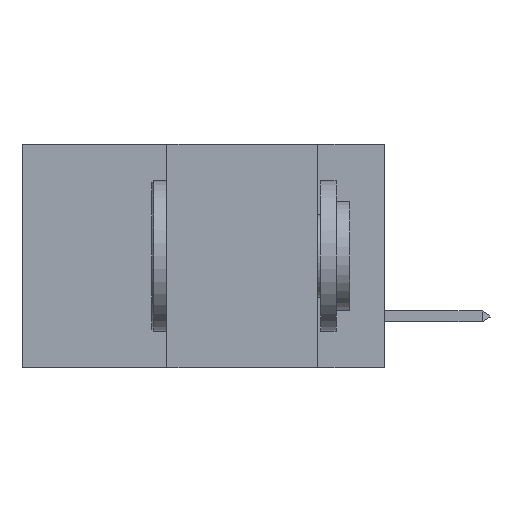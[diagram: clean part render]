
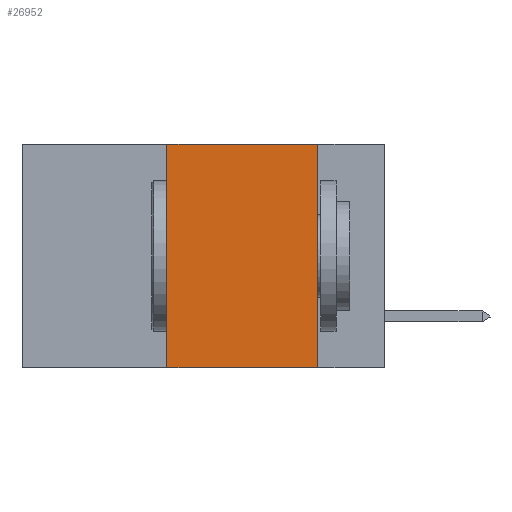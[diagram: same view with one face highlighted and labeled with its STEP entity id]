
A CAD part, left-side view. The second image highlights one B-rep face of the part: STEP entity #26952.
In plain terms, the highlighted planar face has unit normal (-1, 0, 0).
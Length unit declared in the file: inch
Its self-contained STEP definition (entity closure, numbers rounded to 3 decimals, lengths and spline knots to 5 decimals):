
#34 = EDGE_CURVE ( 'NONE', #44070, #2648, #2830, .T. ) ;
#351 = LINE ( 'NONE', #17322, #23861 ) ;
#598 = ORIENTED_EDGE ( 'NONE', *, *, #30831, .F. ) ;
#2648 = VERTEX_POINT ( 'NONE', #30350 ) ;
#2830 = LINE ( 'NONE', #42293, #42597 ) ;
#2924 = DIRECTION ( 'NONE',  ( 1., 0., 0. ) ) ;
#6303 = EDGE_CURVE ( 'NONE', #29232, #2648, #351, .T. ) ;
#7140 = DIRECTION ( 'NONE',  ( 0., 0., -1. ) ) ;
#9015 = ORIENTED_EDGE ( 'NONE', *, *, #34, .F. ) ;
#9149 = CARTESIAN_POINT ( 'NONE',  ( 0., 0.36, 0. ) ) ;
#11955 = FACE_OUTER_BOUND ( 'NONE', #38855, .T. ) ;
#13648 = CARTESIAN_POINT ( 'NONE',  ( 0., 0.36, 0. ) ) ;
#14920 = CARTESIAN_POINT ( 'NONE',  ( 0., 0.36, -0.37 ) ) ;
#17322 = CARTESIAN_POINT ( 'NONE',  ( 0., 0.6, -0.37 ) ) ;
#21343 = DIRECTION ( 'NONE',  ( 0., -1., 0. ) ) ;
#21453 = CARTESIAN_POINT ( 'NONE',  ( 0., 0.6, 0. ) ) ;
#22094 = PLANE ( 'NONE',  #35613 ) ;
#22651 = CARTESIAN_POINT ( 'NONE',  ( 0., 0.11, 0. ) ) ;
#23861 = VECTOR ( 'NONE', #21343, 39.37008 ) ;
#24878 = VECTOR ( 'NONE', #33259, 39.37008 ) ;
#25992 = CARTESIAN_POINT ( 'NONE',  ( 0., 0.6, 0. ) ) ;
#26289 = DIRECTION ( 'NONE',  ( 0., 0., -1. ) ) ;
#26952 = ADVANCED_FACE ( 'NONE', ( #11955 ), #22094, .F. ) ;
#29232 = VERTEX_POINT ( 'NONE', #14920 ) ;
#30350 = CARTESIAN_POINT ( 'NONE',  ( 0., 0.11, -0.37 ) ) ;
#30831 = EDGE_CURVE ( 'NONE', #39962, #44070, #35675, .T. ) ;
#31560 = ORIENTED_EDGE ( 'NONE', *, *, #6303, .T. ) ;
#31675 = VECTOR ( 'NONE', #33351, 39.37008 ) ;
#33259 = DIRECTION ( 'NONE',  ( 0., -1., 0. ) ) ;
#33351 = DIRECTION ( 'NONE',  ( 0., 0., 1. ) ) ;
#35613 = AXIS2_PLACEMENT_3D ( 'NONE', #25992, #2924, #7140 ) ;
#35675 = LINE ( 'NONE', #21453, #24878 ) ;
#36117 = ORIENTED_EDGE ( 'NONE', *, *, #40064, .F. ) ;
#38855 = EDGE_LOOP ( 'NONE', ( #9015, #598, #36117, #31560 ) ) ;
#39478 = LINE ( 'NONE', #13648, #31675 ) ;
#39962 = VERTEX_POINT ( 'NONE', #9149 ) ;
#40064 = EDGE_CURVE ( 'NONE', #29232, #39962, #39478, .T. ) ;
#42293 = CARTESIAN_POINT ( 'NONE',  ( 0., 0.11, 0. ) ) ;
#42597 = VECTOR ( 'NONE', #26289, 39.37008 ) ;
#44070 = VERTEX_POINT ( 'NONE', #22651 ) ;
